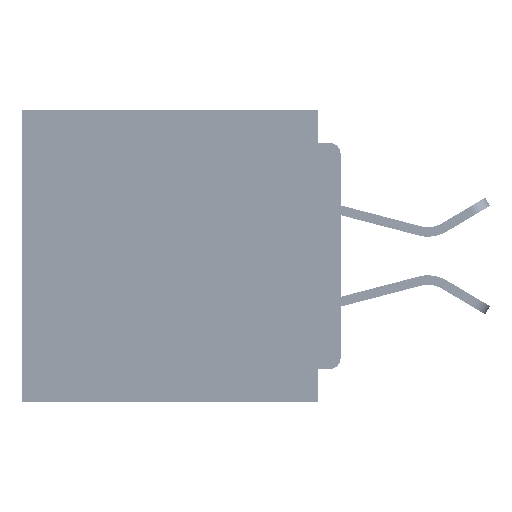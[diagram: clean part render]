
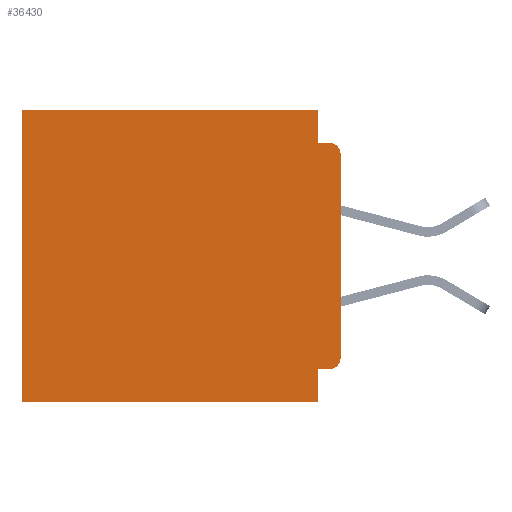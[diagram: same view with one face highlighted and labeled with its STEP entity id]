
A CAD part, left-side view. The second image highlights one B-rep face of the part: STEP entity #36430.
In plain terms, the highlighted planar face has unit normal (-1, 0, 0).
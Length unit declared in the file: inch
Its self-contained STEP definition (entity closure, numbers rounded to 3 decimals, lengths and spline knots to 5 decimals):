
#22 = ORIENTED_EDGE ( 'NONE', *, *, #43413, .F. ) ;
#359 = DIRECTION ( 'NONE',  ( 0., 0., -1. ) ) ;
#789 = LINE ( 'NONE', #23091, #12298 ) ;
#834 = CIRCLE ( 'NONE', #16157, 0.015 ) ;
#1104 = DIRECTION ( 'NONE',  ( 1., 0., 0. ) ) ;
#1120 = DIRECTION ( 'NONE',  ( -1., 0., 0. ) ) ;
#1587 = CARTESIAN_POINT ( 'NONE',  ( 0.3, 0., -0.045 ) ) ;
#1947 = VECTOR ( 'NONE', #44052, 39.37008 ) ;
#2591 = EDGE_LOOP ( 'NONE', ( #22, #35470, #62025, #40396, #23722, #15311, #2999, #9058, #57054, #51496 ) ) ;
#2999 = ORIENTED_EDGE ( 'NONE', *, *, #33760, .F. ) ;
#3796 = LINE ( 'NONE', #19076, #41168 ) ;
#3908 = VECTOR ( 'NONE', #9879, 39.37008 ) ;
#3964 = CARTESIAN_POINT ( 'NONE',  ( 0.3, 0.031, -0.355 ) ) ;
#4649 = EDGE_CURVE ( 'NONE', #36166, #46555, #45424, .T. ) ;
#5063 = CARTESIAN_POINT ( 'NONE',  ( 0.3, 0., -0.4 ) ) ;
#5865 = VERTEX_POINT ( 'NONE', #24933 ) ;
#6940 = EDGE_CURVE ( 'NONE', #49526, #36166, #16919, .T. ) ;
#8636 = CARTESIAN_POINT ( 'NONE',  ( 0.3, 0.031, -0.045 ) ) ;
#9058 = ORIENTED_EDGE ( 'NONE', *, *, #18521, .F. ) ;
#9879 = DIRECTION ( 'NONE',  ( 0., 0., -1. ) ) ;
#10005 = CARTESIAN_POINT ( 'NONE',  ( 0.3, 0.015, -0.34 ) ) ;
#10734 = PLANE ( 'NONE',  #31938 ) ;
#11664 = CARTESIAN_POINT ( 'NONE',  ( 0.3, 0.031, -0.4 ) ) ;
#12298 = VECTOR ( 'NONE', #61794, 39.37008 ) ;
#12398 = EDGE_CURVE ( 'NONE', #60810, #46555, #53549, .T. ) ;
#13510 = EDGE_CURVE ( 'NONE', #57570, #59001, #834, .T. ) ;
#13615 = AXIS2_PLACEMENT_3D ( 'NONE', #30390, #1120, #35304 ) ;
#14911 = DIRECTION ( 'NONE',  ( 0., 0., -1. ) ) ;
#15311 = ORIENTED_EDGE ( 'NONE', *, *, #61375, .T. ) ;
#16157 = AXIS2_PLACEMENT_3D ( 'NONE', #10005, #44073, #14911 ) ;
#16648 = VERTEX_POINT ( 'NONE', #51563 ) ;
#16919 = LINE ( 'NONE', #29334, #3908 ) ;
#18521 = EDGE_CURVE ( 'NONE', #39815, #22611, #789, .T. ) ;
#19076 = CARTESIAN_POINT ( 'NONE',  ( 0.3, 0., -0.355 ) ) ;
#19323 = DIRECTION ( 'NONE',  ( 0., 0., -1. ) ) ;
#19974 = DIRECTION ( 'NONE',  ( 0., 1., 0. ) ) ;
#21381 = CARTESIAN_POINT ( 'NONE',  ( 0.3, 0.015, -0.045 ) ) ;
#21416 = CARTESIAN_POINT ( 'NONE',  ( 0.3, 0., -0.34 ) ) ;
#22611 = VERTEX_POINT ( 'NONE', #11664 ) ;
#23091 = CARTESIAN_POINT ( 'NONE',  ( 0.3, 0.031, -0.4 ) ) ;
#23722 = ORIENTED_EDGE ( 'NONE', *, *, #35764, .T. ) ;
#24025 = DIRECTION ( 'NONE',  ( 0., 1., 0. ) ) ;
#24933 = CARTESIAN_POINT ( 'NONE',  ( 0.3, 0.437, -0.4 ) ) ;
#29334 = CARTESIAN_POINT ( 'NONE',  ( 0.3, 0.031, 0. ) ) ;
#29537 = CARTESIAN_POINT ( 'NONE',  ( 0.3, 0.031, 0. ) ) ;
#30377 = CARTESIAN_POINT ( 'NONE',  ( 0.3, 0., -0.4 ) ) ;
#30390 = CARTESIAN_POINT ( 'NONE',  ( 0.3, 0.015, -0.06 ) ) ;
#31313 = LINE ( 'NONE', #34524, #55506 ) ;
#31347 = VECTOR ( 'NONE', #19323, 39.37008 ) ;
#31938 = AXIS2_PLACEMENT_3D ( 'NONE', #30377, #1104, #35291 ) ;
#32556 = VECTOR ( 'NONE', #45470, 39.37008 ) ;
#33760 = EDGE_CURVE ( 'NONE', #22611, #5865, #55189, .T. ) ;
#33762 = FACE_OUTER_BOUND ( 'NONE', #2591, .T. ) ;
#34524 = CARTESIAN_POINT ( 'NONE',  ( 0.3, 0.437, -0.4 ) ) ;
#35291 = DIRECTION ( 'NONE',  ( 0., 0., -1. ) ) ;
#35304 = DIRECTION ( 'NONE',  ( 0., 0., -1. ) ) ;
#35470 = ORIENTED_EDGE ( 'NONE', *, *, #12398, .T. ) ;
#35764 = EDGE_CURVE ( 'NONE', #49526, #16648, #62370, .T. ) ;
#36166 = VERTEX_POINT ( 'NONE', #8636 ) ;
#36430 = ADVANCED_FACE ( 'NONE', ( #33762 ), #10734, .F. ) ;
#39815 = VERTEX_POINT ( 'NONE', #3964 ) ;
#40396 = ORIENTED_EDGE ( 'NONE', *, *, #6940, .F. ) ;
#41168 = VECTOR ( 'NONE', #24025, 39.37008 ) ;
#43413 = EDGE_CURVE ( 'NONE', #60810, #59001, #57036, .T. ) ;
#44052 = DIRECTION ( 'NONE',  ( 0., 1., 0. ) ) ;
#44073 = DIRECTION ( 'NONE',  ( -1., 0., 0. ) ) ;
#44240 = CARTESIAN_POINT ( 'NONE',  ( 0.3, 0., 0. ) ) ;
#45424 = LINE ( 'NONE', #1587, #32556 ) ;
#45470 = DIRECTION ( 'NONE',  ( 0., -1., 0. ) ) ;
#46555 = VERTEX_POINT ( 'NONE', #21381 ) ;
#48474 = CARTESIAN_POINT ( 'NONE',  ( 0.3, 0., -0.4 ) ) ;
#49190 = CARTESIAN_POINT ( 'NONE',  ( 0.3, 0., -0.06 ) ) ;
#49526 = VERTEX_POINT ( 'NONE', #29537 ) ;
#49665 = VECTOR ( 'NONE', #19974, 39.37008 ) ;
#51496 = ORIENTED_EDGE ( 'NONE', *, *, #13510, .T. ) ;
#51563 = CARTESIAN_POINT ( 'NONE',  ( 0.3, 0.437, 0. ) ) ;
#53549 = CIRCLE ( 'NONE', #13615, 0.015 ) ;
#55189 = LINE ( 'NONE', #5063, #1947 ) ;
#55506 = VECTOR ( 'NONE', #359, 39.37008 ) ;
#56835 = EDGE_CURVE ( 'NONE', #57570, #39815, #3796, .T. ) ;
#57036 = LINE ( 'NONE', #48474, #31347 ) ;
#57054 = ORIENTED_EDGE ( 'NONE', *, *, #56835, .F. ) ;
#57570 = VERTEX_POINT ( 'NONE', #59059 ) ;
#59001 = VERTEX_POINT ( 'NONE', #21416 ) ;
#59059 = CARTESIAN_POINT ( 'NONE',  ( 0.3, 0.015, -0.355 ) ) ;
#60810 = VERTEX_POINT ( 'NONE', #49190 ) ;
#61375 = EDGE_CURVE ( 'NONE', #16648, #5865, #31313, .T. ) ;
#61794 = DIRECTION ( 'NONE',  ( 0., 0., -1. ) ) ;
#62025 = ORIENTED_EDGE ( 'NONE', *, *, #4649, .F. ) ;
#62370 = LINE ( 'NONE', #44240, #49665 ) ;
